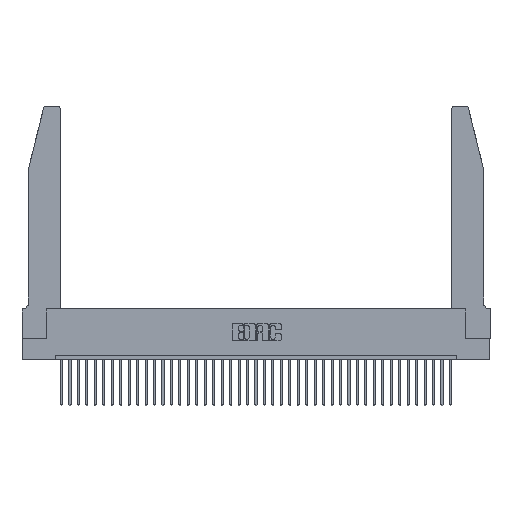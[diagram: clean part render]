
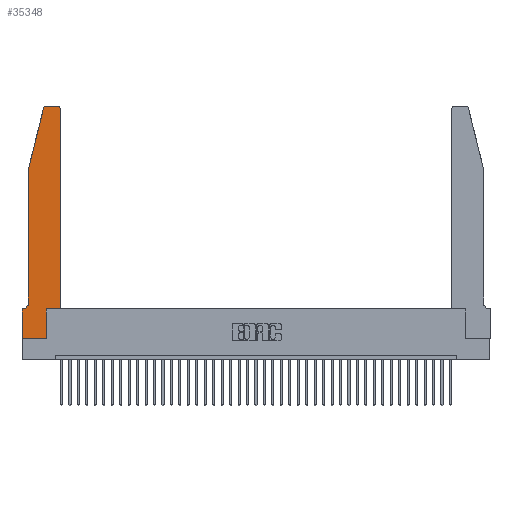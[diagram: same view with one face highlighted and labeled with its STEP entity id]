
A CAD part, top view. The second image highlights one B-rep face of the part: STEP entity #35348.
In plain terms, the highlighted planar face has unit normal (0, 0, 1).
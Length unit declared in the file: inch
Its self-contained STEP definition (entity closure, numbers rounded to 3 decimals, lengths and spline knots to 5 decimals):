
#373 = DIRECTION ( 'NONE',  ( 0., -1., 0. ) ) ;
#731 = VERTEX_POINT ( 'NONE', #33612 ) ;
#1391 = CARTESIAN_POINT ( 'NONE',  ( 0.4505, 0.35, 0.37 ) ) ;
#1439 = LINE ( 'NONE', #6999, #9558 ) ;
#1553 = DIRECTION ( 'NONE',  ( 1., 0., 0. ) ) ;
#1903 = VERTEX_POINT ( 'NONE', #37546 ) ;
#2823 = DIRECTION ( 'NONE',  ( 0., 0., 1. ) ) ;
#2848 = CARTESIAN_POINT ( 'NONE',  ( 0.4505, 0.35, 0.37 ) ) ;
#2882 = LINE ( 'NONE', #18669, #7756 ) ;
#3300 = CARTESIAN_POINT ( 'NONE',  ( 0.2865, 0.35, 0.37 ) ) ;
#3353 = DIRECTION ( 'NONE',  ( 1., 0., 0. ) ) ;
#3393 = CARTESIAN_POINT ( 'NONE',  ( 0.0755, 0.42, 0.37 ) ) ;
#3469 = CIRCLE ( 'NONE', #19171, 0.03 ) ;
#3886 = CARTESIAN_POINT ( 'NONE',  ( 0.2605, 2.75, 0.37 ) ) ;
#4555 = VECTOR ( 'NONE', #30973, 39.37008 ) ;
#4650 = LINE ( 'NONE', #21081, #28095 ) ;
#4951 = LINE ( 'NONE', #35396, #7861 ) ;
#6791 = ORIENTED_EDGE ( 'NONE', *, *, #7222, .T. ) ;
#6841 = CARTESIAN_POINT ( 'NONE',  ( 0., 0., 0.37 ) ) ;
#6999 = CARTESIAN_POINT ( 'NONE',  ( 0.4505, 0.35, 0.37 ) ) ;
#7046 = ORIENTED_EDGE ( 'NONE', *, *, #37641, .T. ) ;
#7222 = EDGE_CURVE ( 'NONE', #17807, #31539, #28948, .T. ) ;
#7249 = AXIS2_PLACEMENT_3D ( 'NONE', #33255, #2823, #24221 ) ;
#7342 = ORIENTED_EDGE ( 'NONE', *, *, #34952, .T. ) ;
#7719 = CARTESIAN_POINT ( 'NONE',  ( 0.0055, 0.42, 0.37 ) ) ;
#7756 = VECTOR ( 'NONE', #373, 39.37008 ) ;
#7861 = VECTOR ( 'NONE', #22931, 39.37008 ) ;
#7950 = LINE ( 'NONE', #1391, #32267 ) ;
#8924 = DIRECTION ( 'NONE',  ( -1., 0., 0. ) ) ;
#8948 = EDGE_CURVE ( 'NONE', #12360, #17807, #23265, .T. ) ;
#9558 = VECTOR ( 'NONE', #3353, 39.37008 ) ;
#9595 = LINE ( 'NONE', #11910, #24433 ) ;
#10132 = DIRECTION ( 'NONE',  ( 0., 0., 1. ) ) ;
#10485 = VERTEX_POINT ( 'NONE', #27127 ) ;
#10742 = DIRECTION ( 'NONE',  ( 0., 0., -1. ) ) ;
#11084 = DIRECTION ( 'NONE',  ( 0., -1., 0. ) ) ;
#11910 = CARTESIAN_POINT ( 'NONE',  ( 0.2865, 0.35, 0.37 ) ) ;
#11990 = VECTOR ( 'NONE', #31509, 39.37008 ) ;
#12360 = VERTEX_POINT ( 'NONE', #28958 ) ;
#12760 = ORIENTED_EDGE ( 'NONE', *, *, #36437, .T. ) ;
#12905 = VERTEX_POINT ( 'NONE', #24771 ) ;
#13240 = PLANE ( 'NONE',  #31552 ) ;
#13329 = ORIENTED_EDGE ( 'NONE', *, *, #32018, .T. ) ;
#13431 = VERTEX_POINT ( 'NONE', #28041 ) ;
#13854 = DIRECTION ( 'NONE',  ( -1., 0., 0. ) ) ;
#15016 = DIRECTION ( 'NONE',  ( 0., 1., 0. ) ) ;
#17790 = EDGE_CURVE ( 'NONE', #26259, #731, #28052, .T. ) ;
#17807 = VERTEX_POINT ( 'NONE', #22927 ) ;
#18040 = VERTEX_POINT ( 'NONE', #2848 ) ;
#18669 = CARTESIAN_POINT ( 'NONE',  ( 0.0755, 2., 0.37 ) ) ;
#19024 = EDGE_CURVE ( 'NONE', #18040, #1903, #7950, .T. ) ;
#19171 = AXIS2_PLACEMENT_3D ( 'NONE', #35273, #25643, #1553 ) ;
#19206 = EDGE_LOOP ( 'NONE', ( #31765, #34423, #7342, #13329, #24197, #29090, #23090, #6791, #23228, #7046, #36720, #12760 ) ) ;
#20134 = LINE ( 'NONE', #3886, #11990 ) ;
#21081 = CARTESIAN_POINT ( 'NONE',  ( 0.0755, 0.35, 0.37 ) ) ;
#22191 = CARTESIAN_POINT ( 'NONE',  ( 0., 0.35, 0.37 ) ) ;
#22431 = EDGE_CURVE ( 'NONE', #731, #12360, #4650, .T. ) ;
#22704 = DIRECTION ( 'NONE',  ( 1., 0., 0. ) ) ;
#22927 = CARTESIAN_POINT ( 'NONE',  ( 0., 0., 0.37 ) ) ;
#22931 = DIRECTION ( 'NONE',  ( -0.239, -0.971, 0. ) ) ;
#23090 = ORIENTED_EDGE ( 'NONE', *, *, #8948, .T. ) ;
#23228 = ORIENTED_EDGE ( 'NONE', *, *, #37527, .T. ) ;
#23265 = LINE ( 'NONE', #35344, #38448 ) ;
#23626 = VERTEX_POINT ( 'NONE', #26779 ) ;
#24197 = ORIENTED_EDGE ( 'NONE', *, *, #17790, .T. ) ;
#24221 = DIRECTION ( 'NONE',  ( 1., 0., 0. ) ) ;
#24433 = VECTOR ( 'NONE', #15016, 39.37008 ) ;
#24771 = CARTESIAN_POINT ( 'NONE',  ( 0.4205, 2.75, 0.37 ) ) ;
#25643 = DIRECTION ( 'NONE',  ( 0., 0., 1. ) ) ;
#26259 = VERTEX_POINT ( 'NONE', #3393 ) ;
#26779 = CARTESIAN_POINT ( 'NONE',  ( 0.25487, 2.72718, 0.37 ) ) ;
#26891 = EDGE_CURVE ( 'NONE', #12905, #13431, #20134, .T. ) ;
#27127 = CARTESIAN_POINT ( 'NONE',  ( 0.0755, 2., 0.37 ) ) ;
#28041 = CARTESIAN_POINT ( 'NONE',  ( 0.284, 2.75, 0.37 ) ) ;
#28052 = CIRCLE ( 'NONE', #30155, 0.07 ) ;
#28095 = VECTOR ( 'NONE', #8924, 39.37008 ) ;
#28948 = LINE ( 'NONE', #6841, #4555 ) ;
#28958 = CARTESIAN_POINT ( 'NONE',  ( 0., 0.35, 0.37 ) ) ;
#29090 = ORIENTED_EDGE ( 'NONE', *, *, #22431, .T. ) ;
#29185 = DIRECTION ( 'NONE',  ( 0., 1., 0. ) ) ;
#30155 = AXIS2_PLACEMENT_3D ( 'NONE', #7719, #10742, #13854 ) ;
#30262 = FACE_OUTER_BOUND ( 'NONE', #19206, .T. ) ;
#30973 = DIRECTION ( 'NONE',  ( 1., 0., 0. ) ) ;
#31509 = DIRECTION ( 'NONE',  ( -1., 0., 0. ) ) ;
#31539 = VERTEX_POINT ( 'NONE', #39442 ) ;
#31552 = AXIS2_PLACEMENT_3D ( 'NONE', #22191, #10132, #22704 ) ;
#31765 = ORIENTED_EDGE ( 'NONE', *, *, #26891, .T. ) ;
#32018 = EDGE_CURVE ( 'NONE', #10485, #26259, #2882, .T. ) ;
#32267 = VECTOR ( 'NONE', #29185, 39.37008 ) ;
#33255 = CARTESIAN_POINT ( 'NONE',  ( 0.284, 2.72, 0.37 ) ) ;
#33612 = CARTESIAN_POINT ( 'NONE',  ( 0.0055, 0.35, 0.37 ) ) ;
#33876 = EDGE_CURVE ( 'NONE', #13431, #23626, #39066, .T. ) ;
#34423 = ORIENTED_EDGE ( 'NONE', *, *, #33876, .T. ) ;
#34952 = EDGE_CURVE ( 'NONE', #23626, #10485, #4951, .T. ) ;
#35273 = CARTESIAN_POINT ( 'NONE',  ( 0.4205, 2.72, 0.37 ) ) ;
#35344 = CARTESIAN_POINT ( 'NONE',  ( 0., 0., 0.37 ) ) ;
#35348 = ADVANCED_FACE ( 'NONE', ( #30262 ), #13240, .T. ) ;
#35396 = CARTESIAN_POINT ( 'NONE',  ( 0.0755, 2., 0.37 ) ) ;
#36437 = EDGE_CURVE ( 'NONE', #1903, #12905, #3469, .T. ) ;
#36720 = ORIENTED_EDGE ( 'NONE', *, *, #19024, .T. ) ;
#37527 = EDGE_CURVE ( 'NONE', #31539, #38193, #9595, .T. ) ;
#37546 = CARTESIAN_POINT ( 'NONE',  ( 0.4505, 2.72, 0.37 ) ) ;
#37641 = EDGE_CURVE ( 'NONE', #38193, #18040, #1439, .T. ) ;
#38193 = VERTEX_POINT ( 'NONE', #3300 ) ;
#38448 = VECTOR ( 'NONE', #11084, 39.37008 ) ;
#39066 = CIRCLE ( 'NONE', #7249, 0.03 ) ;
#39442 = CARTESIAN_POINT ( 'NONE',  ( 0.2865, 0., 0.37 ) ) ;
